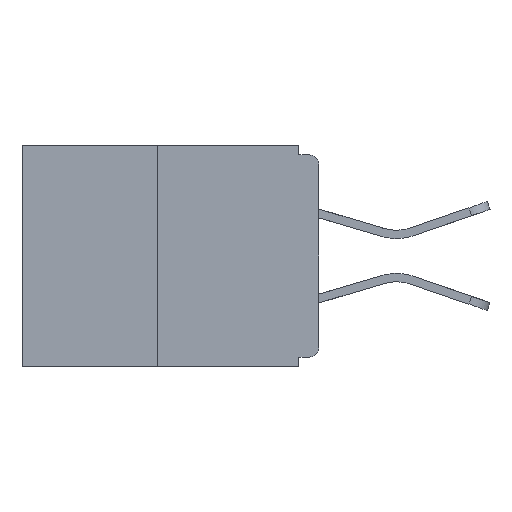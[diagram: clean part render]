
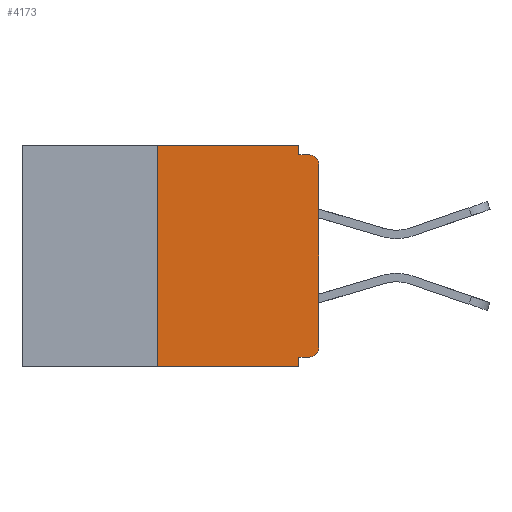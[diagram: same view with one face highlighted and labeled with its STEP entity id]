
A CAD part, left-side view. The second image highlights one B-rep face of the part: STEP entity #4173.
In plain terms, the highlighted planar face has unit normal (-1, 0, 0).
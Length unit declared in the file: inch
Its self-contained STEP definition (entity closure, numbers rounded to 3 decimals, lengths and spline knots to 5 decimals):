
#91 = DIRECTION ( 'NONE',  ( 0., 0., 1. ) ) ;
#119 = AXIS2_PLACEMENT_3D ( 'NONE', #6289, #9748, #389 ) ;
#187 = CARTESIAN_POINT ( 'NONE',  ( 0., 0.015, -0.03 ) ) ;
#201 = VERTEX_POINT ( 'NONE', #9122 ) ;
#256 = DIRECTION ( 'NONE',  ( -1., 0., 0. ) ) ;
#352 = CARTESIAN_POINT ( 'NONE',  ( 0., 0., -0.015 ) ) ;
#389 = DIRECTION ( 'NONE',  ( 0., 0., -1. ) ) ;
#487 = CARTESIAN_POINT ( 'NONE',  ( 0., 0.031, -0.343 ) ) ;
#627 = ORIENTED_EDGE ( 'NONE', *, *, #3494, .T. ) ;
#690 = CARTESIAN_POINT ( 'NONE',  ( 0., 0.031, -0.328 ) ) ;
#699 = EDGE_CURVE ( 'NONE', #1846, #13898, #2505, .T. ) ;
#1027 = PLANE ( 'NONE',  #13279 ) ;
#1117 = VERTEX_POINT ( 'NONE', #8186 ) ;
#1519 = EDGE_CURVE ( 'NONE', #11214, #7610, #4908, .T. ) ;
#1837 = ORIENTED_EDGE ( 'NONE', *, *, #13170, .T. ) ;
#1846 = VERTEX_POINT ( 'NONE', #6161 ) ;
#2099 = VERTEX_POINT ( 'NONE', #13861 ) ;
#2436 = DIRECTION ( 'NONE',  ( 0., -1., 0. ) ) ;
#2505 = LINE ( 'NONE', #12479, #7203 ) ;
#2594 = ORIENTED_EDGE ( 'NONE', *, *, #3098, .F. ) ;
#2619 = CARTESIAN_POINT ( 'NONE',  ( 0., 0.031, 0. ) ) ;
#2718 = LINE ( 'NONE', #3837, #13748 ) ;
#2997 = CARTESIAN_POINT ( 'NONE',  ( 0., 0.46, -0.343 ) ) ;
#3007 = FACE_OUTER_BOUND ( 'NONE', #7511, .T. ) ;
#3098 = EDGE_CURVE ( 'NONE', #3547, #1117, #8367, .T. ) ;
#3313 = CARTESIAN_POINT ( 'NONE',  ( 0., 0., -0.03 ) ) ;
#3316 = DIRECTION ( 'NONE',  ( 0., 0., 1. ) ) ;
#3494 = EDGE_CURVE ( 'NONE', #11993, #1117, #5848, .T. ) ;
#3547 = VERTEX_POINT ( 'NONE', #11659 ) ;
#3807 = LINE ( 'NONE', #8542, #12749 ) ;
#3837 = CARTESIAN_POINT ( 'NONE',  ( 0., 0., -0.328 ) ) ;
#4173 = ADVANCED_FACE ( 'NONE', ( #3007 ), #1027, .F. ) ;
#4743 = DIRECTION ( 'NONE',  ( 0., 0., -1. ) ) ;
#4908 = LINE ( 'NONE', #487, #5722 ) ;
#5119 = DIRECTION ( 'NONE',  ( 0., 1., 0. ) ) ;
#5481 = LINE ( 'NONE', #14699, #11729 ) ;
#5722 = VECTOR ( 'NONE', #9486, 39.37008 ) ;
#5848 = CIRCLE ( 'NONE', #6560, 0.015 ) ;
#5855 = LINE ( 'NONE', #2619, #9601 ) ;
#6161 = CARTESIAN_POINT ( 'NONE',  ( 0., 0.25, -0.343 ) ) ;
#6289 = CARTESIAN_POINT ( 'NONE',  ( 0., 0.015, -0.313 ) ) ;
#6560 = AXIS2_PLACEMENT_3D ( 'NONE', #187, #256, #4743 ) ;
#6725 = CARTESIAN_POINT ( 'NONE',  ( 0., 0.46, 0. ) ) ;
#7203 = VECTOR ( 'NONE', #3316, 39.37008 ) ;
#7225 = EDGE_CURVE ( 'NONE', #9444, #2099, #8007, .T. ) ;
#7305 = VECTOR ( 'NONE', #11093, 39.37008 ) ;
#7409 = DIRECTION ( 'NONE',  ( 0., -1., 0. ) ) ;
#7511 = EDGE_LOOP ( 'NONE', ( #12787, #10537, #7915, #8347, #14687, #12996, #1837, #627, #2594, #13346 ) ) ;
#7558 = EDGE_CURVE ( 'NONE', #1846, #7610, #8348, .T. ) ;
#7571 = DIRECTION ( 'NONE',  ( 0., 0., -1. ) ) ;
#7610 = VERTEX_POINT ( 'NONE', #11790 ) ;
#7915 = ORIENTED_EDGE ( 'NONE', *, *, #7558, .T. ) ;
#8007 = CIRCLE ( 'NONE', #119, 0.015 ) ;
#8186 = CARTESIAN_POINT ( 'NONE',  ( 0., 0.015, -0.015 ) ) ;
#8347 = ORIENTED_EDGE ( 'NONE', *, *, #1519, .F. ) ;
#8348 = LINE ( 'NONE', #2997, #7305 ) ;
#8367 = LINE ( 'NONE', #352, #8780 ) ;
#8542 = CARTESIAN_POINT ( 'NONE',  ( 0., 0.46, 0. ) ) ;
#8780 = VECTOR ( 'NONE', #2436, 39.37008 ) ;
#8948 = EDGE_CURVE ( 'NONE', #9444, #11214, #2718, .T. ) ;
#9122 = CARTESIAN_POINT ( 'NONE',  ( 0., 0.031, 0. ) ) ;
#9444 = VERTEX_POINT ( 'NONE', #13178 ) ;
#9486 = DIRECTION ( 'NONE',  ( 0., 0., -1. ) ) ;
#9601 = VECTOR ( 'NONE', #10437, 39.37008 ) ;
#9748 = DIRECTION ( 'NONE',  ( -1., 0., 0. ) ) ;
#10437 = DIRECTION ( 'NONE',  ( 0., 0., -1. ) ) ;
#10537 = ORIENTED_EDGE ( 'NONE', *, *, #699, .F. ) ;
#11093 = DIRECTION ( 'NONE',  ( 0., -1., 0. ) ) ;
#11214 = VERTEX_POINT ( 'NONE', #690 ) ;
#11616 = EDGE_CURVE ( 'NONE', #13898, #201, #3807, .T. ) ;
#11659 = CARTESIAN_POINT ( 'NONE',  ( 0., 0.031, -0.015 ) ) ;
#11729 = VECTOR ( 'NONE', #91, 39.37008 ) ;
#11790 = CARTESIAN_POINT ( 'NONE',  ( 0., 0.031, -0.343 ) ) ;
#11993 = VERTEX_POINT ( 'NONE', #3313 ) ;
#12211 = DIRECTION ( 'NONE',  ( 1., 0., 0. ) ) ;
#12479 = CARTESIAN_POINT ( 'NONE',  ( 0., 0.25, 0. ) ) ;
#12749 = VECTOR ( 'NONE', #7409, 39.37008 ) ;
#12787 = ORIENTED_EDGE ( 'NONE', *, *, #11616, .F. ) ;
#12996 = ORIENTED_EDGE ( 'NONE', *, *, #7225, .T. ) ;
#13170 = EDGE_CURVE ( 'NONE', #2099, #11993, #5481, .T. ) ;
#13178 = CARTESIAN_POINT ( 'NONE',  ( 0., 0.015, -0.328 ) ) ;
#13279 = AXIS2_PLACEMENT_3D ( 'NONE', #6725, #12211, #7571 ) ;
#13346 = ORIENTED_EDGE ( 'NONE', *, *, #13803, .F. ) ;
#13748 = VECTOR ( 'NONE', #5119, 39.37008 ) ;
#13803 = EDGE_CURVE ( 'NONE', #201, #3547, #5855, .T. ) ;
#13861 = CARTESIAN_POINT ( 'NONE',  ( 0., 0., -0.313 ) ) ;
#13898 = VERTEX_POINT ( 'NONE', #14316 ) ;
#14316 = CARTESIAN_POINT ( 'NONE',  ( 0., 0.25, 0. ) ) ;
#14687 = ORIENTED_EDGE ( 'NONE', *, *, #8948, .F. ) ;
#14699 = CARTESIAN_POINT ( 'NONE',  ( 0., 0., 0. ) ) ;
